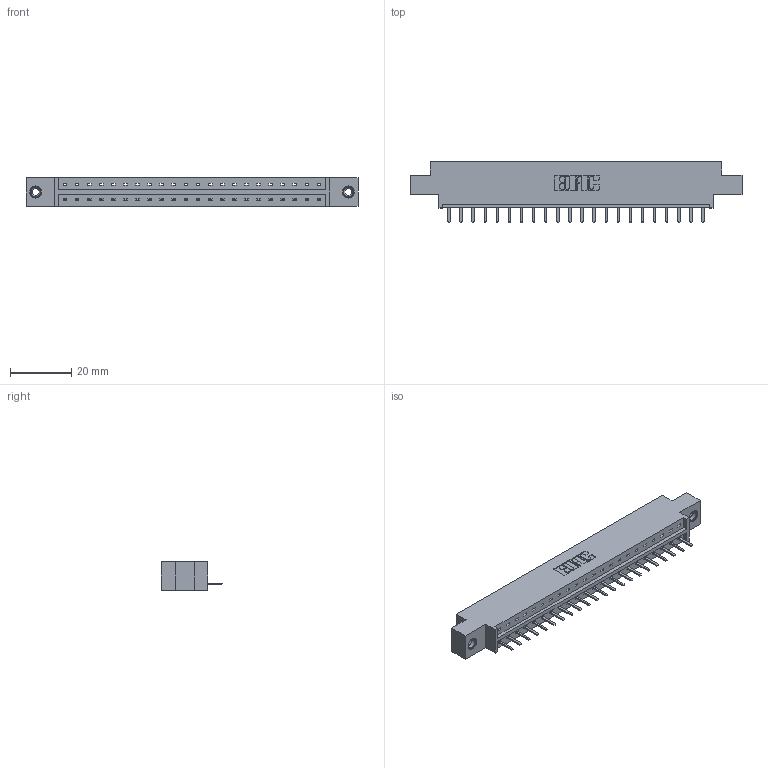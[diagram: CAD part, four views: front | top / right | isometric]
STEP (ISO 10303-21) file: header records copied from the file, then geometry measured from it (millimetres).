
FILE_DESCRIPTION (( 'STEP AP203' ), '1' );
FILE_NAME ('333-022-520-608.STEP', '2018-08-02T01:40:31', ( '' ), ( '' ), 'SwSTEP 2.0', 'SolidWorks 2016', '' );
FILE_SCHEMA (( 'CONFIG_CONTROL_DESIGN' ));
Length unit declared in the file: inch
Products named in the file (4): 333 Part_Offset - .156 Dia - TI; 345-292-001_345-293-120; 345-250-001_345-250-003-102; 333-022-520-608
Assembly tree (25 placements, depth 2):
  333-022-520-608
    333 Part_Offset - .156 Dia - TI
    345-292-001_345-293-120  x22
    345-250-001_345-250-003-102  x2
Bounding box: 108.71 x 20.02 x 9.4 mm (x, y, z)
Volume: 10469.9 mm3; surface area: 11199.2 mm2
Topology: 25 solids, 25 shells, 1542 faces, 4507 edges, 2938 vertices
Faces by surface type: plane 1074, cylinder 452, cone 12, torus 4
Entity records: 17468 total; most frequent: CARTESIAN_POINT 3011, ORIENTED_EDGE 2950, DIRECTION 2601, EDGE_CURVE 1475, LINE 1323, VECTOR 1323, VERTEX_POINT 976, AXIS2_PLACEMENT_3D 639
